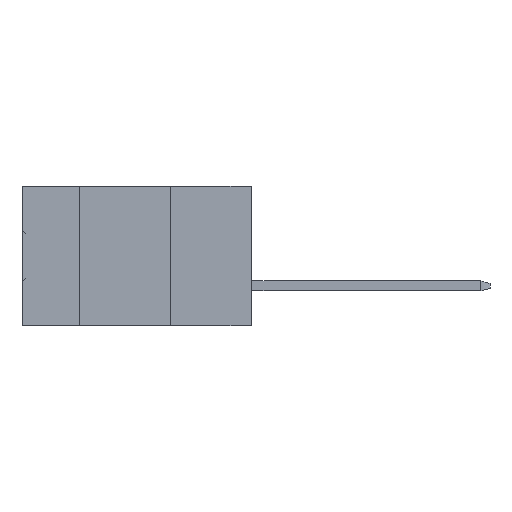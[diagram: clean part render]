
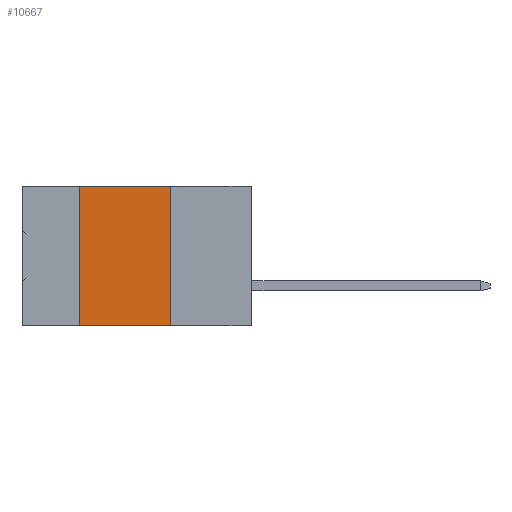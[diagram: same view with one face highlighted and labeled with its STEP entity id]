
A CAD part, left-side view. The second image highlights one B-rep face of the part: STEP entity #10667.
In plain terms, the highlighted planar face has unit normal (-1, 0, 0).
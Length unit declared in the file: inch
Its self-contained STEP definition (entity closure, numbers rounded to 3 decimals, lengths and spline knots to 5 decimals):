
#307 = VERTEX_POINT ( 'NONE', #7835 ) ;
#1567 = DIRECTION ( 'NONE',  ( 0., 0., -1. ) ) ;
#1754 = LINE ( 'NONE', #6283, #15489 ) ;
#1913 = ORIENTED_EDGE ( 'NONE', *, *, #10646, .T. ) ;
#3153 = ORIENTED_EDGE ( 'NONE', *, *, #6820, .F. ) ;
#3838 = LINE ( 'NONE', #28598, #12604 ) ;
#4447 = DIRECTION ( 'NONE',  ( 0., 0., 1. ) ) ;
#5817 = AXIS2_PLACEMENT_3D ( 'NONE', #17758, #29365, #1567 ) ;
#6283 = CARTESIAN_POINT ( 'NONE',  ( 0., 0.72, 0. ) ) ;
#6687 = ORIENTED_EDGE ( 'NONE', *, *, #10350, .F. ) ;
#6820 = EDGE_CURVE ( 'NONE', #14038, #17929, #25150, .T. ) ;
#6942 = FACE_OUTER_BOUND ( 'NONE', #22671, .T. ) ;
#7835 = CARTESIAN_POINT ( 'NONE',  ( 0., 0.254, 0. ) ) ;
#7841 = DIRECTION ( 'NONE',  ( 0., 0., -1. ) ) ;
#10350 = EDGE_CURVE ( 'NONE', #17929, #307, #1754, .T. ) ;
#10646 = EDGE_CURVE ( 'NONE', #14038, #16013, #3838, .T. ) ;
#10667 = ADVANCED_FACE ( 'NONE', ( #6942 ), #18445, .F. ) ;
#12131 = CARTESIAN_POINT ( 'NONE',  ( 0., 0.254, -0.437 ) ) ;
#12604 = VECTOR ( 'NONE', #24080, 39.37008 ) ;
#14038 = VERTEX_POINT ( 'NONE', #18225 ) ;
#15489 = VECTOR ( 'NONE', #20346, 39.37008 ) ;
#16013 = VERTEX_POINT ( 'NONE', #12131 ) ;
#16497 = LINE ( 'NONE', #19056, #22039 ) ;
#17758 = CARTESIAN_POINT ( 'NONE',  ( 0., 0.72, 0. ) ) ;
#17929 = VERTEX_POINT ( 'NONE', #18486 ) ;
#18225 = CARTESIAN_POINT ( 'NONE',  ( 0., 0.54, -0.437 ) ) ;
#18445 = PLANE ( 'NONE',  #5817 ) ;
#18486 = CARTESIAN_POINT ( 'NONE',  ( 0., 0.54, 0. ) ) ;
#19056 = CARTESIAN_POINT ( 'NONE',  ( 0., 0.254, -0.437 ) ) ;
#19657 = EDGE_CURVE ( 'NONE', #307, #16013, #16497, .T. ) ;
#20346 = DIRECTION ( 'NONE',  ( 0., -1., 0. ) ) ;
#20788 = CARTESIAN_POINT ( 'NONE',  ( 0., 0.54, -0.437 ) ) ;
#21002 = ORIENTED_EDGE ( 'NONE', *, *, #19657, .F. ) ;
#22039 = VECTOR ( 'NONE', #7841, 39.37008 ) ;
#22671 = EDGE_LOOP ( 'NONE', ( #21002, #6687, #3153, #1913 ) ) ;
#24080 = DIRECTION ( 'NONE',  ( 0., -1., 0. ) ) ;
#25150 = LINE ( 'NONE', #20788, #28365 ) ;
#28365 = VECTOR ( 'NONE', #4447, 39.37008 ) ;
#28598 = CARTESIAN_POINT ( 'NONE',  ( 0., 0.72, -0.437 ) ) ;
#29365 = DIRECTION ( 'NONE',  ( 1., 0., 0. ) ) ;
